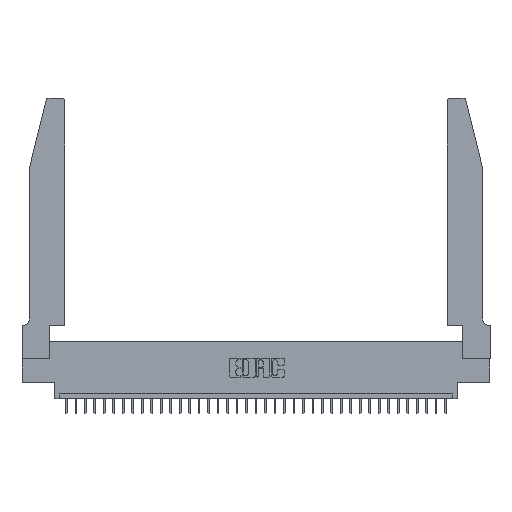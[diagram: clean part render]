
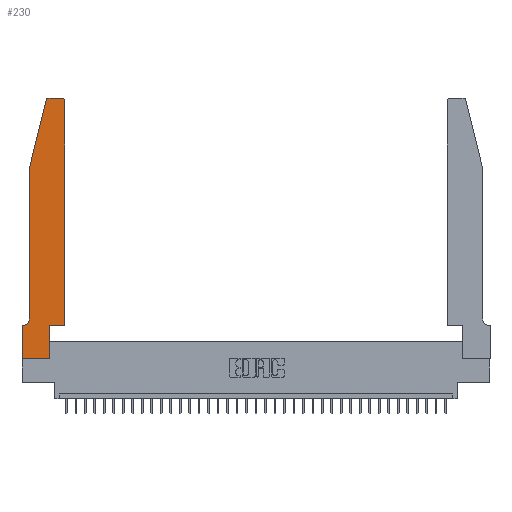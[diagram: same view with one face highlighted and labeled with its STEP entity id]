
A CAD part, top view. The second image highlights one B-rep face of the part: STEP entity #230.
In plain terms, the highlighted planar face has unit normal (0, 0, 1).
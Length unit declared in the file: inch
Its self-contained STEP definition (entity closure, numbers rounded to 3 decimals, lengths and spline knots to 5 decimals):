
#21 = CARTESIAN_POINT ( 'NONE',  ( 0.4505, 0.35, 0.37 ) ) ;
#230 = ADVANCED_FACE ( 'NONE', ( #24167 ), #27860, .T. ) ;
#1151 = EDGE_CURVE ( 'NONE', #21200, #3809, #7193, .T. ) ;
#1392 = CARTESIAN_POINT ( 'NONE',  ( 0., 0.35, 0.37 ) ) ;
#1621 = ORIENTED_EDGE ( 'NONE', *, *, #16474, .T. ) ;
#1979 = VERTEX_POINT ( 'NONE', #19665 ) ;
#2092 = ORIENTED_EDGE ( 'NONE', *, *, #14137, .T. ) ;
#2733 = LINE ( 'NONE', #26747, #17488 ) ;
#3809 = VERTEX_POINT ( 'NONE', #20934 ) ;
#4487 = DIRECTION ( 'NONE',  ( 1., 0., 0. ) ) ;
#4571 = ORIENTED_EDGE ( 'NONE', *, *, #27574, .T. ) ;
#5030 = CARTESIAN_POINT ( 'NONE',  ( 0.0755, 0.42, 0.37 ) ) ;
#5039 = DIRECTION ( 'NONE',  ( 0., 0., -1. ) ) ;
#5187 = VECTOR ( 'NONE', #15507, 39.37008 ) ;
#6056 = CIRCLE ( 'NONE', #24090, 0.03 ) ;
#6291 = EDGE_CURVE ( 'NONE', #1979, #14787, #12476, .T. ) ;
#6769 = EDGE_CURVE ( 'NONE', #20985, #1979, #17695, .T. ) ;
#7193 = LINE ( 'NONE', #21, #27137 ) ;
#8036 = CARTESIAN_POINT ( 'NONE',  ( 0.2865, 0., 0.37 ) ) ;
#8204 = CARTESIAN_POINT ( 'NONE',  ( 0., 0., 0.37 ) ) ;
#8394 = AXIS2_PLACEMENT_3D ( 'NONE', #30621, #14050, #19641 ) ;
#8523 = CARTESIAN_POINT ( 'NONE',  ( 0.4505, 0.35, 0.37 ) ) ;
#9021 = VECTOR ( 'NONE', #28912, 39.37008 ) ;
#9179 = CARTESIAN_POINT ( 'NONE',  ( 0.0755, 2., 0.37 ) ) ;
#9403 = DIRECTION ( 'NONE',  ( -0.239, -0.971, 0. ) ) ;
#9447 = VECTOR ( 'NONE', #9403, 39.37008 ) ;
#10115 = CARTESIAN_POINT ( 'NONE',  ( 0.284, 2.72, 0.37 ) ) ;
#10499 = CARTESIAN_POINT ( 'NONE',  ( 0.4205, 2.75, 0.37 ) ) ;
#11634 = VERTEX_POINT ( 'NONE', #8204 ) ;
#11661 = ORIENTED_EDGE ( 'NONE', *, *, #21554, .T. ) ;
#12343 = VERTEX_POINT ( 'NONE', #13488 ) ;
#12476 = LINE ( 'NONE', #24712, #35867 ) ;
#13145 = EDGE_CURVE ( 'NONE', #14787, #19388, #33036, .T. ) ;
#13276 = DIRECTION ( 'NONE',  ( -1., 0., 0. ) ) ;
#13488 = CARTESIAN_POINT ( 'NONE',  ( 0.284, 2.75, 0.37 ) ) ;
#13700 = ORIENTED_EDGE ( 'NONE', *, *, #30135, .T. ) ;
#14050 = DIRECTION ( 'NONE',  ( 0., 0., 1. ) ) ;
#14137 = EDGE_CURVE ( 'NONE', #3809, #20370, #23022, .T. ) ;
#14448 = ORIENTED_EDGE ( 'NONE', *, *, #6291, .T. ) ;
#14486 = ORIENTED_EDGE ( 'NONE', *, *, #13145, .T. ) ;
#14787 = VERTEX_POINT ( 'NONE', #5030 ) ;
#15193 = CARTESIAN_POINT ( 'NONE',  ( 0., 0., 0.37 ) ) ;
#15507 = DIRECTION ( 'NONE',  ( -1., 0., 0. ) ) ;
#15689 = DIRECTION ( 'NONE',  ( 0., 0., 1. ) ) ;
#16474 = EDGE_CURVE ( 'NONE', #11634, #21010, #25488, .T. ) ;
#16731 = VECTOR ( 'NONE', #34704, 39.37008 ) ;
#17236 = ORIENTED_EDGE ( 'NONE', *, *, #6769, .T. ) ;
#17488 = VECTOR ( 'NONE', #18537, 39.37008 ) ;
#17660 = CARTESIAN_POINT ( 'NONE',  ( 0., 0., 0.37 ) ) ;
#17695 = LINE ( 'NONE', #9179, #9447 ) ;
#18537 = DIRECTION ( 'NONE',  ( 1., 0., 0. ) ) ;
#18737 = DIRECTION ( 'NONE',  ( -1., 0., 0. ) ) ;
#19388 = VERTEX_POINT ( 'NONE', #31960 ) ;
#19641 = DIRECTION ( 'NONE',  ( 1., 0., 0. ) ) ;
#19665 = CARTESIAN_POINT ( 'NONE',  ( 0.0755, 2., 0.37 ) ) ;
#20001 = CARTESIAN_POINT ( 'NONE',  ( 0.2865, 0.35, 0.37 ) ) ;
#20370 = VERTEX_POINT ( 'NONE', #10499 ) ;
#20934 = CARTESIAN_POINT ( 'NONE',  ( 0.4505, 2.72, 0.37 ) ) ;
#20985 = VERTEX_POINT ( 'NONE', #30072 ) ;
#21010 = VERTEX_POINT ( 'NONE', #8036 ) ;
#21090 = DIRECTION ( 'NONE',  ( 0., 0., 1. ) ) ;
#21200 = VERTEX_POINT ( 'NONE', #8523 ) ;
#21300 = EDGE_CURVE ( 'NONE', #21010, #22049, #23806, .T. ) ;
#21554 = EDGE_CURVE ( 'NONE', #19388, #32007, #27288, .T. ) ;
#22049 = VERTEX_POINT ( 'NONE', #20001 ) ;
#22194 = EDGE_LOOP ( 'NONE', ( #30238, #13700, #17236, #14448, #14486, #11661, #30151, #1621, #25860, #4571, #31198, #2092 ) ) ;
#23022 = CIRCLE ( 'NONE', #23295, 0.03 ) ;
#23295 = AXIS2_PLACEMENT_3D ( 'NONE', #29672, #21090, #4487 ) ;
#23711 = VECTOR ( 'NONE', #18737, 39.37008 ) ;
#23806 = LINE ( 'NONE', #33729, #25104 ) ;
#24090 = AXIS2_PLACEMENT_3D ( 'NONE', #10115, #15689, #32403 ) ;
#24167 = FACE_OUTER_BOUND ( 'NONE', #22194, .T. ) ;
#24214 = CARTESIAN_POINT ( 'NONE',  ( 0.0755, 0.35, 0.37 ) ) ;
#24550 = EDGE_CURVE ( 'NONE', #20370, #12343, #33717, .T. ) ;
#24712 = CARTESIAN_POINT ( 'NONE',  ( 0.0755, 2., 0.37 ) ) ;
#25104 = VECTOR ( 'NONE', #31164, 39.37008 ) ;
#25488 = LINE ( 'NONE', #17660, #9021 ) ;
#25860 = ORIENTED_EDGE ( 'NONE', *, *, #21300, .T. ) ;
#26747 = CARTESIAN_POINT ( 'NONE',  ( 0.4505, 0.35, 0.37 ) ) ;
#27137 = VECTOR ( 'NONE', #30312, 39.37008 ) ;
#27203 = AXIS2_PLACEMENT_3D ( 'NONE', #35702, #5039, #13276 ) ;
#27288 = LINE ( 'NONE', #24214, #5187 ) ;
#27574 = EDGE_CURVE ( 'NONE', #22049, #21200, #2733, .T. ) ;
#27860 = PLANE ( 'NONE',  #8394 ) ;
#28912 = DIRECTION ( 'NONE',  ( 1., 0., 0. ) ) ;
#29672 = CARTESIAN_POINT ( 'NONE',  ( 0.4205, 2.72, 0.37 ) ) ;
#30072 = CARTESIAN_POINT ( 'NONE',  ( 0.25487, 2.72718, 0.37 ) ) ;
#30135 = EDGE_CURVE ( 'NONE', #12343, #20985, #6056, .T. ) ;
#30151 = ORIENTED_EDGE ( 'NONE', *, *, #32843, .T. ) ;
#30238 = ORIENTED_EDGE ( 'NONE', *, *, #24550, .T. ) ;
#30312 = DIRECTION ( 'NONE',  ( 0., 1., 0. ) ) ;
#30621 = CARTESIAN_POINT ( 'NONE',  ( 0., 0.35, 0.37 ) ) ;
#31164 = DIRECTION ( 'NONE',  ( 0., 1., 0. ) ) ;
#31198 = ORIENTED_EDGE ( 'NONE', *, *, #1151, .T. ) ;
#31960 = CARTESIAN_POINT ( 'NONE',  ( 0.0055, 0.35, 0.37 ) ) ;
#32007 = VERTEX_POINT ( 'NONE', #1392 ) ;
#32403 = DIRECTION ( 'NONE',  ( 1., 0., 0. ) ) ;
#32843 = EDGE_CURVE ( 'NONE', #32007, #11634, #33201, .T. ) ;
#33036 = CIRCLE ( 'NONE', #27203, 0.07 ) ;
#33201 = LINE ( 'NONE', #15193, #16731 ) ;
#33717 = LINE ( 'NONE', #34741, #23711 ) ;
#33729 = CARTESIAN_POINT ( 'NONE',  ( 0.2865, 0.35, 0.37 ) ) ;
#34704 = DIRECTION ( 'NONE',  ( 0., -1., 0. ) ) ;
#34741 = CARTESIAN_POINT ( 'NONE',  ( 0.2605, 2.75, 0.37 ) ) ;
#35032 = DIRECTION ( 'NONE',  ( 0., -1., 0. ) ) ;
#35702 = CARTESIAN_POINT ( 'NONE',  ( 0.0055, 0.42, 0.37 ) ) ;
#35867 = VECTOR ( 'NONE', #35032, 39.37008 ) ;
